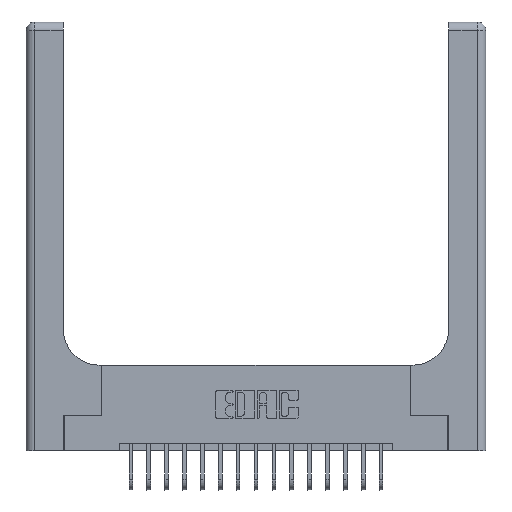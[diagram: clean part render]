
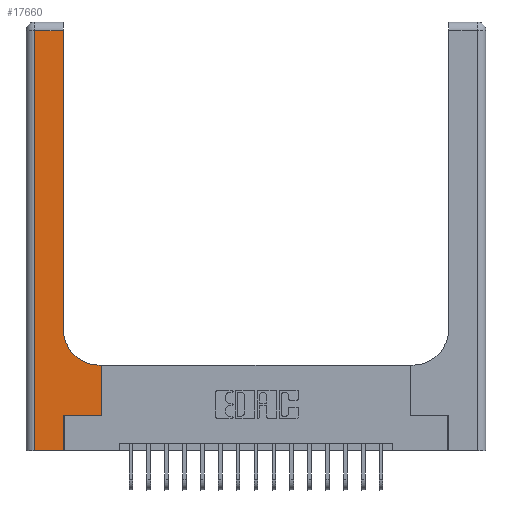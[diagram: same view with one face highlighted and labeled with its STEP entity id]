
A CAD part, top view. The second image highlights one B-rep face of the part: STEP entity #17660.
In plain terms, the highlighted planar face has unit normal (0, 0, 1).
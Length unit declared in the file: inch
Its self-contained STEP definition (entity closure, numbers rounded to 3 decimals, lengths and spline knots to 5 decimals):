
#237 = EDGE_CURVE ( 'NONE', #10433, #1933, #10204, .T. ) ;
#518 = EDGE_LOOP ( 'NONE', ( #2331, #6421, #5729, #5080, #4287, #8609, #3204, #766, #18017 ) ) ;
#766 = ORIENTED_EDGE ( 'NONE', *, *, #10390, .T. ) ;
#922 = CARTESIAN_POINT ( 'NONE',  ( 0.51, 0.6, 0.37 ) ) ;
#1479 = DIRECTION ( 'NONE',  ( 1., 0., 0. ) ) ;
#1664 = CARTESIAN_POINT ( 'NONE',  ( 0.51, 0.85, 0.37 ) ) ;
#1933 = VERTEX_POINT ( 'NONE', #5836 ) ;
#2145 = CARTESIAN_POINT ( 'NONE',  ( 0.26, 0.6, 0.37 ) ) ;
#2331 = ORIENTED_EDGE ( 'NONE', *, *, #4217, .T. ) ;
#2624 = CARTESIAN_POINT ( 'NONE',  ( 0.265, 0.25, 0.37 ) ) ;
#3156 = VERTEX_POINT ( 'NONE', #2624 ) ;
#3204 = ORIENTED_EDGE ( 'NONE', *, *, #9987, .T. ) ;
#3319 = CARTESIAN_POINT ( 'NONE',  ( 0.26, 2.94, 0.37 ) ) ;
#3568 = PLANE ( 'NONE',  #3649 ) ;
#3617 = DIRECTION ( 'NONE',  ( 1., 0., 0. ) ) ;
#3649 = AXIS2_PLACEMENT_3D ( 'NONE', #12600, #12061, #18366 ) ;
#3833 = CARTESIAN_POINT ( 'NONE',  ( 0.06, 2.94, 0.37 ) ) ;
#3896 = VECTOR ( 'NONE', #12591, 39.37008 ) ;
#4217 = EDGE_CURVE ( 'NONE', #1933, #17274, #14373, .T. ) ;
#4287 = ORIENTED_EDGE ( 'NONE', *, *, #8278, .T. ) ;
#4540 = EDGE_CURVE ( 'NONE', #15737, #18393, #8848, .T. ) ;
#4677 = CARTESIAN_POINT ( 'NONE',  ( 0.06, 0., 0.37 ) ) ;
#5056 = CARTESIAN_POINT ( 'NONE',  ( 0.265, 0.25, 0.37 ) ) ;
#5080 = ORIENTED_EDGE ( 'NONE', *, *, #8641, .T. ) ;
#5330 = DIRECTION ( 'NONE',  ( 0., 1., 0. ) ) ;
#5338 = LINE ( 'NONE', #5056, #18435 ) ;
#5458 = FACE_OUTER_BOUND ( 'NONE', #518, .T. ) ;
#5729 = ORIENTED_EDGE ( 'NONE', *, *, #4540, .T. ) ;
#5836 = CARTESIAN_POINT ( 'NONE',  ( 0.26, 0.85, 0.37 ) ) ;
#6029 = DIRECTION ( 'NONE',  ( 1., 0., 0. ) ) ;
#6421 = ORIENTED_EDGE ( 'NONE', *, *, #8861, .T. ) ;
#7168 = CARTESIAN_POINT ( 'NONE',  ( 0., 0., 0.37 ) ) ;
#7443 = DIRECTION ( 'NONE',  ( 0., 0., -1. ) ) ;
#8278 = EDGE_CURVE ( 'NONE', #10546, #3156, #14164, .T. ) ;
#8329 = VERTEX_POINT ( 'NONE', #17282 ) ;
#8570 = DIRECTION ( 'NONE',  ( 0., 1., 0. ) ) ;
#8609 = ORIENTED_EDGE ( 'NONE', *, *, #16942, .T. ) ;
#8641 = EDGE_CURVE ( 'NONE', #18393, #10546, #11318, .T. ) ;
#8848 = LINE ( 'NONE', #10343, #16370 ) ;
#8861 = EDGE_CURVE ( 'NONE', #17274, #15737, #9397, .T. ) ;
#9397 = LINE ( 'NONE', #9490, #3896 ) ;
#9424 = DIRECTION ( 'NONE',  ( -1., 0., 0. ) ) ;
#9490 = CARTESIAN_POINT ( 'NONE',  ( 0., 2.94, 0.37 ) ) ;
#9697 = VECTOR ( 'NONE', #9424, 39.37008 ) ;
#9824 = CARTESIAN_POINT ( 'NONE',  ( 0.528, 0.6, 0.37 ) ) ;
#9973 = DIRECTION ( 'NONE',  ( 0., -1., 0. ) ) ;
#9987 = EDGE_CURVE ( 'NONE', #8329, #11198, #18507, .T. ) ;
#10010 = DIRECTION ( 'NONE',  ( 0., 1., 0. ) ) ;
#10039 = VECTOR ( 'NONE', #10010, 39.37008 ) ;
#10204 = CIRCLE ( 'NONE', #11704, 0.25 ) ;
#10343 = CARTESIAN_POINT ( 'NONE',  ( 0.06, 3., 0.37 ) ) ;
#10390 = EDGE_CURVE ( 'NONE', #11198, #10433, #15055, .T. ) ;
#10433 = VERTEX_POINT ( 'NONE', #922 ) ;
#10546 = VERTEX_POINT ( 'NONE', #14646 ) ;
#11198 = VERTEX_POINT ( 'NONE', #9824 ) ;
#11318 = LINE ( 'NONE', #7168, #13893 ) ;
#11571 = VECTOR ( 'NONE', #8570, 39.37008 ) ;
#11704 = AXIS2_PLACEMENT_3D ( 'NONE', #1664, #7443, #6029 ) ;
#12061 = DIRECTION ( 'NONE',  ( 0., 0., -1. ) ) ;
#12591 = DIRECTION ( 'NONE',  ( -1., 0., 0. ) ) ;
#12600 = CARTESIAN_POINT ( 'NONE',  ( 0., 3., 0.37 ) ) ;
#13281 = VECTOR ( 'NONE', #5330, 39.37008 ) ;
#13893 = VECTOR ( 'NONE', #1479, 39.37008 ) ;
#14164 = LINE ( 'NONE', #15767, #13281 ) ;
#14373 = LINE ( 'NONE', #15794, #11571 ) ;
#14646 = CARTESIAN_POINT ( 'NONE',  ( 0.265, 0., 0.37 ) ) ;
#15055 = LINE ( 'NONE', #2145, #9697 ) ;
#15737 = VERTEX_POINT ( 'NONE', #3833 ) ;
#15767 = CARTESIAN_POINT ( 'NONE',  ( 0.265, 0., 0.37 ) ) ;
#15794 = CARTESIAN_POINT ( 'NONE',  ( 0.26, 3., 0.37 ) ) ;
#16370 = VECTOR ( 'NONE', #9973, 39.37008 ) ;
#16942 = EDGE_CURVE ( 'NONE', #3156, #8329, #5338, .T. ) ;
#16992 = CARTESIAN_POINT ( 'NONE',  ( 0.528, 0.25, 0.37 ) ) ;
#17274 = VERTEX_POINT ( 'NONE', #3319 ) ;
#17282 = CARTESIAN_POINT ( 'NONE',  ( 0.528, 0.25, 0.37 ) ) ;
#17660 = ADVANCED_FACE ( 'NONE', ( #5458 ), #3568, .F. ) ;
#18017 = ORIENTED_EDGE ( 'NONE', *, *, #237, .T. ) ;
#18366 = DIRECTION ( 'NONE',  ( -1., 0., 0. ) ) ;
#18393 = VERTEX_POINT ( 'NONE', #4677 ) ;
#18435 = VECTOR ( 'NONE', #3617, 39.37008 ) ;
#18507 = LINE ( 'NONE', #16992, #10039 ) ;
